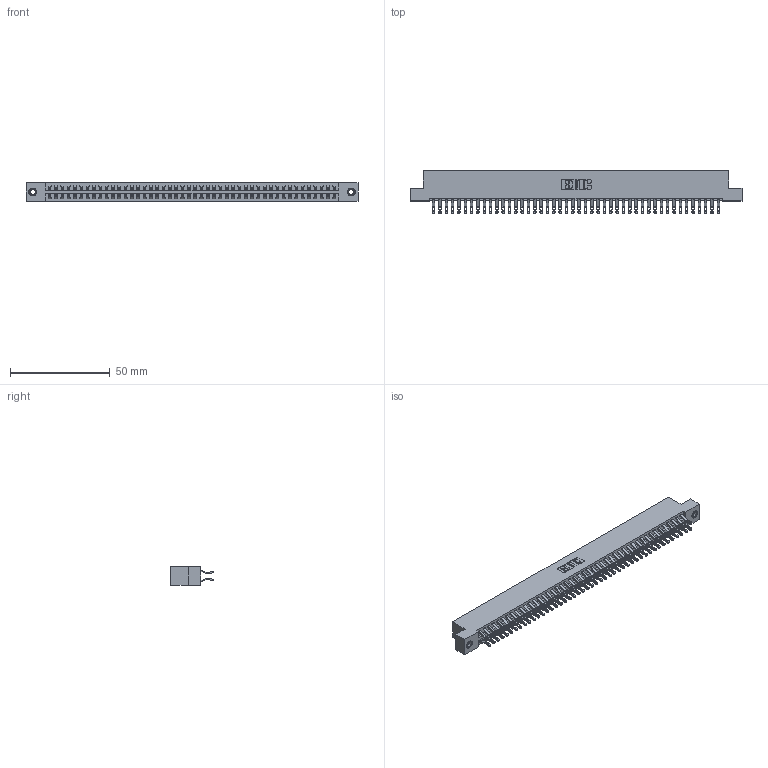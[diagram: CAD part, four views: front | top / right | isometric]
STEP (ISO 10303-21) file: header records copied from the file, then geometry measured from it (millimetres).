
FILE_DESCRIPTION (( 'STEP AP203' ), '1' );
FILE_NAME ('346-092-555-207.STEP', '2022-05-26T07:41:17', ( '' ), ( '' ), 'SwSTEP 2.0', 'SolidWorks 2020', '' );
FILE_SCHEMA (( 'CONFIG_CONTROL_DESIGN' ));
Length unit declared in the file: inch
Products named in the file (4): 346-092-555-207; 346 Part_Flush Mounting Lugs - 0.156 Dia-TI; 345-250-001_345-250-005-103; 345-292-001_555 Tail
Assembly tree (95 placements, depth 2):
  346-092-555-207
    346 Part_Flush Mounting Lugs - 0.156 Dia-TI
    345-292-001_555 Tail  x92
    345-250-001_345-250-005-103  x2
Bounding box: 166.62 x 21.46 x 9.4 mm (x, y, z)
Volume: 16532.3 mm3; surface area: 23772.6 mm2
Topology: 95 solids, 95 shells, 5518 faces, 17301 edges, 11526 vertices
Faces by surface type: plane 3144, cylinder 2358, cone 12, torus 4
Entity records: 30994 total; most frequent: CARTESIAN_POINT 5121, ORIENTED_EDGE 5018, DIRECTION 4559, EDGE_CURVE 2509, VECTOR 2153, LINE 2153, VERTEX_POINT 1668, AXIS2_PLACEMENT_3D 1203
